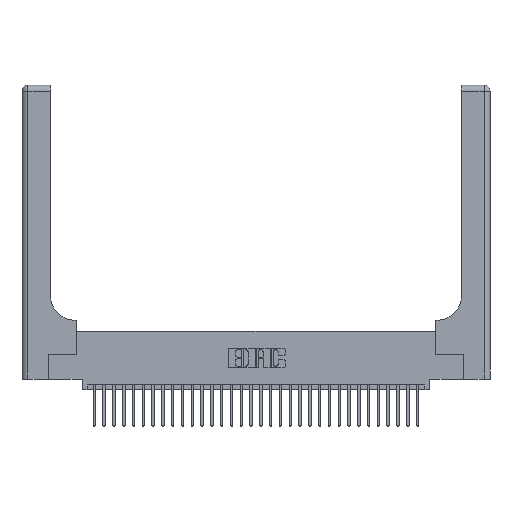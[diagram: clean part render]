
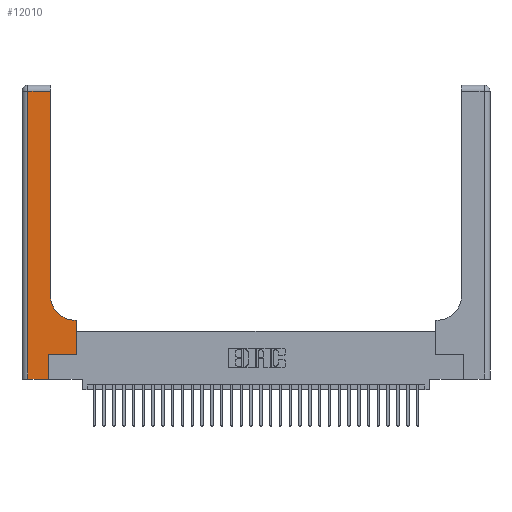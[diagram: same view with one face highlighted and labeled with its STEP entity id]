
A CAD part, top view. The second image highlights one B-rep face of the part: STEP entity #12010.
In plain terms, the highlighted planar face has unit normal (0, 0, 1).
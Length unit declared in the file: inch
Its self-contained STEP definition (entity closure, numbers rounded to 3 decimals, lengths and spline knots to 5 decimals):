
#1607 = AXIS2_PLACEMENT_3D ( 'NONE', #28493, #13227, #30996 ) ;
#2036 = VECTOR ( 'NONE', #19556, 39.37008 ) ;
#2162 = EDGE_CURVE ( 'NONE', #8781, #16737, #29964, .T. ) ;
#2212 = ORIENTED_EDGE ( 'NONE', *, *, #12288, .T. ) ;
#2395 = CARTESIAN_POINT ( 'NONE',  ( 0.269, 0., 0.37 ) ) ;
#4140 = ORIENTED_EDGE ( 'NONE', *, *, #9084, .T. ) ;
#4264 = LINE ( 'NONE', #2395, #17105 ) ;
#4943 = EDGE_CURVE ( 'NONE', #5304, #13113, #11876, .T. ) ;
#4963 = CARTESIAN_POINT ( 'NONE',  ( 0.2915, 3., 0.37 ) ) ;
#5017 = DIRECTION ( 'NONE',  ( 0., 1., 0. ) ) ;
#5215 = EDGE_CURVE ( 'NONE', #16737, #17898, #4264, .T. ) ;
#5304 = VERTEX_POINT ( 'NONE', #23199 ) ;
#6378 = CARTESIAN_POINT ( 'NONE',  ( 0.06, 2.94, 0.37 ) ) ;
#6480 = PLANE ( 'NONE',  #30843 ) ;
#6596 = CARTESIAN_POINT ( 'NONE',  ( 0.06, 3., 0.37 ) ) ;
#6936 = CARTESIAN_POINT ( 'NONE',  ( 0.269, 0.25, 0.37 ) ) ;
#8254 = EDGE_CURVE ( 'NONE', #19769, #5304, #26999, .T. ) ;
#8551 = ORIENTED_EDGE ( 'NONE', *, *, #8254, .T. ) ;
#8781 = VERTEX_POINT ( 'NONE', #25995 ) ;
#8948 = LINE ( 'NONE', #14401, #2036 ) ;
#9084 = EDGE_CURVE ( 'NONE', #16649, #22115, #8948, .T. ) ;
#9118 = DIRECTION ( 'NONE',  ( -1., 0., 0. ) ) ;
#9708 = VERTEX_POINT ( 'NONE', #27232 ) ;
#9879 = ORIENTED_EDGE ( 'NONE', *, *, #18265, .T. ) ;
#10161 = EDGE_CURVE ( 'NONE', #22115, #8781, #26879, .T. ) ;
#10370 = EDGE_LOOP ( 'NONE', ( #2212, #4140, #12404, #17147, #29863, #29773, #8551, #12181, #9879 ) ) ;
#11642 = DIRECTION ( 'NONE',  ( -1., 0., 0. ) ) ;
#11876 = LINE ( 'NONE', #21869, #19488 ) ;
#12010 = ADVANCED_FACE ( 'NONE', ( #14323 ), #6480, .F. ) ;
#12181 = ORIENTED_EDGE ( 'NONE', *, *, #4943, .T. ) ;
#12288 = EDGE_CURVE ( 'NONE', #9708, #16649, #25960, .T. ) ;
#12404 = ORIENTED_EDGE ( 'NONE', *, *, #10161, .T. ) ;
#12719 = DIRECTION ( 'NONE',  ( 0., 1., 0. ) ) ;
#13113 = VERTEX_POINT ( 'NONE', #13156 ) ;
#13156 = CARTESIAN_POINT ( 'NONE',  ( 0.5415, 0.6, 0.37 ) ) ;
#13227 = DIRECTION ( 'NONE',  ( 0., 0., -1. ) ) ;
#13393 = VECTOR ( 'NONE', #28844, 39.37008 ) ;
#14064 = EDGE_CURVE ( 'NONE', #17898, #19769, #30340, .T. ) ;
#14100 = CARTESIAN_POINT ( 'NONE',  ( 0.5585, 0.25, 0.37 ) ) ;
#14323 = FACE_OUTER_BOUND ( 'NONE', #10370, .T. ) ;
#14401 = CARTESIAN_POINT ( 'NONE',  ( 0., 2.94, 0.37 ) ) ;
#16489 = CARTESIAN_POINT ( 'NONE',  ( 0.269, 0.25, 0.37 ) ) ;
#16649 = VERTEX_POINT ( 'NONE', #32049 ) ;
#16737 = VERTEX_POINT ( 'NONE', #27381 ) ;
#17105 = VECTOR ( 'NONE', #5017, 39.37008 ) ;
#17147 = ORIENTED_EDGE ( 'NONE', *, *, #2162, .T. ) ;
#17898 = VERTEX_POINT ( 'NONE', #16489 ) ;
#18265 = EDGE_CURVE ( 'NONE', #13113, #9708, #32779, .T. ) ;
#19488 = VECTOR ( 'NONE', #9118, 39.37008 ) ;
#19556 = DIRECTION ( 'NONE',  ( -1., 0., 0. ) ) ;
#19769 = VERTEX_POINT ( 'NONE', #14100 ) ;
#21869 = CARTESIAN_POINT ( 'NONE',  ( 0.2915, 0.6, 0.37 ) ) ;
#21933 = DIRECTION ( 'NONE',  ( 0., -1., 0. ) ) ;
#22115 = VERTEX_POINT ( 'NONE', #6378 ) ;
#22484 = VECTOR ( 'NONE', #26630, 39.37008 ) ;
#23199 = CARTESIAN_POINT ( 'NONE',  ( 0.5585, 0.6, 0.37 ) ) ;
#24096 = CARTESIAN_POINT ( 'NONE',  ( 0., 0., 0.37 ) ) ;
#24431 = CARTESIAN_POINT ( 'NONE',  ( 0., 3., 0.37 ) ) ;
#25960 = LINE ( 'NONE', #4963, #31778 ) ;
#25995 = CARTESIAN_POINT ( 'NONE',  ( 0.06, 0., 0.37 ) ) ;
#26349 = CARTESIAN_POINT ( 'NONE',  ( 0.5585, 0.25, 0.37 ) ) ;
#26630 = DIRECTION ( 'NONE',  ( 1., 0., 0. ) ) ;
#26879 = LINE ( 'NONE', #6596, #32692 ) ;
#26949 = DIRECTION ( 'NONE',  ( 0., 0., -1. ) ) ;
#26999 = LINE ( 'NONE', #26349, #13393 ) ;
#27232 = CARTESIAN_POINT ( 'NONE',  ( 0.2915, 0.85, 0.37 ) ) ;
#27381 = CARTESIAN_POINT ( 'NONE',  ( 0.269, 0., 0.37 ) ) ;
#27391 = DIRECTION ( 'NONE',  ( 1., 0., 0. ) ) ;
#28493 = CARTESIAN_POINT ( 'NONE',  ( 0.5415, 0.85, 0.37 ) ) ;
#28844 = DIRECTION ( 'NONE',  ( 0., 1., 0. ) ) ;
#29773 = ORIENTED_EDGE ( 'NONE', *, *, #14064, .T. ) ;
#29863 = ORIENTED_EDGE ( 'NONE', *, *, #5215, .T. ) ;
#29964 = LINE ( 'NONE', #24096, #22484 ) ;
#30340 = LINE ( 'NONE', #6936, #31146 ) ;
#30843 = AXIS2_PLACEMENT_3D ( 'NONE', #24431, #26949, #11642 ) ;
#30996 = DIRECTION ( 'NONE',  ( 1., 0., 0. ) ) ;
#31146 = VECTOR ( 'NONE', #27391, 39.37008 ) ;
#31778 = VECTOR ( 'NONE', #12719, 39.37008 ) ;
#32049 = CARTESIAN_POINT ( 'NONE',  ( 0.2915, 2.94, 0.37 ) ) ;
#32692 = VECTOR ( 'NONE', #21933, 39.37008 ) ;
#32779 = CIRCLE ( 'NONE', #1607, 0.25 ) ;
